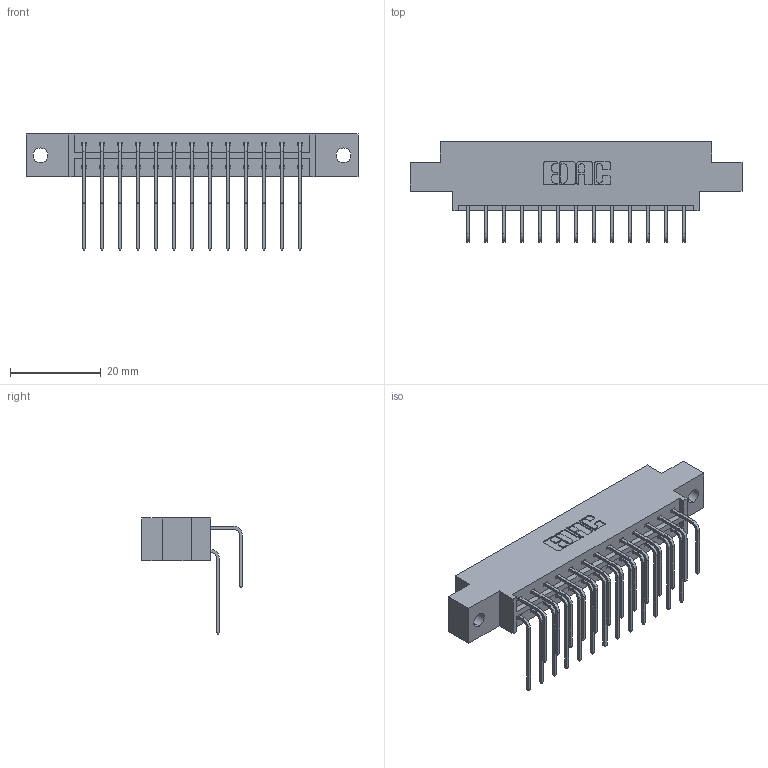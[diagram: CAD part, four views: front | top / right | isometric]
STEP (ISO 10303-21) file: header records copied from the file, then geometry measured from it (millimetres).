
FILE_DESCRIPTION (( 'STEP AP203' ), '1' );
FILE_NAME ('333-026-558-802.STEP', '2018-08-02T13:28:31', ( '' ), ( '' ), 'SwSTEP 2.0', 'SolidWorks 2016', '' );
FILE_SCHEMA (( 'CONFIG_CONTROL_DESIGN' ));
Length unit declared in the file: inch
Products named in the file (4): 333 Part_Offset - .128 Dia; 345-292-001_558 559 Tail - 1; 345-292-001_558 Tail - 2; 333-026-558-802
Assembly tree (27 placements, depth 2):
  333-026-558-802
    333 Part_Offset - .128 Dia
    345-292-001_558 559 Tail - 1  x13
    345-292-001_558 Tail - 2  x13
Bounding box: 73.05 x 22.17 x 25.53 mm (x, y, z)
Volume: 7072.3 mm3; surface area: 8744.2 mm2
Topology: 27 solids, 27 shells, 1522 faces, 4509 edges, 2970 vertices
Faces by surface type: plane 1062, cylinder 460
Entity records: 14033 total; most frequent: CARTESIAN_POINT 2413, ORIENTED_EDGE 2298, DIRECTION 2093, EDGE_CURVE 1149, VECTOR 981, LINE 981, VERTEX_POINT 762, AXIS2_PLACEMENT_3D 556
